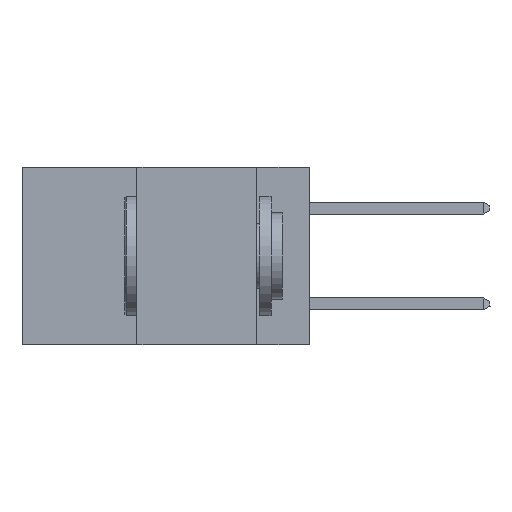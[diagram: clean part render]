
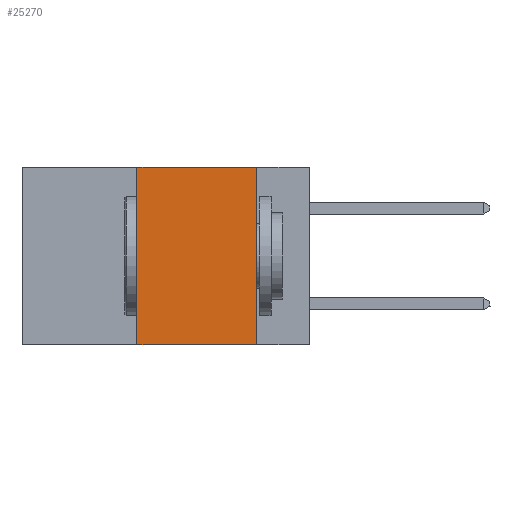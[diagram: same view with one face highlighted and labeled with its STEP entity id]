
A CAD part, left-side view. The second image highlights one B-rep face of the part: STEP entity #25270.
In plain terms, the highlighted planar face has unit normal (-1, 0, 0).
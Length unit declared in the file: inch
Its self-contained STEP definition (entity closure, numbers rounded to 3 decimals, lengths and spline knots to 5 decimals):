
#163 = DIRECTION ( 'NONE',  ( 0., 0., 1. ) ) ;
#1433 = VECTOR ( 'NONE', #27203, 39.37008 ) ;
#1575 = CARTESIAN_POINT ( 'NONE',  ( 0., 0.6, -0.37 ) ) ;
#2614 = ORIENTED_EDGE ( 'NONE', *, *, #15378, .F. ) ;
#3255 = EDGE_CURVE ( 'NONE', #10480, #33487, #26829, .T. ) ;
#4716 = VECTOR ( 'NONE', #163, 39.37008 ) ;
#5505 = FACE_OUTER_BOUND ( 'NONE', #15615, .T. ) ;
#6661 = EDGE_CURVE ( 'NONE', #14457, #33487, #10487, .T. ) ;
#7569 = DIRECTION ( 'NONE',  ( 1., 0., 0. ) ) ;
#8015 = CARTESIAN_POINT ( 'NONE',  ( 0., 0.6, 0. ) ) ;
#8068 = CARTESIAN_POINT ( 'NONE',  ( 0., 0.6, 0. ) ) ;
#10480 = VERTEX_POINT ( 'NONE', #25116 ) ;
#10487 = LINE ( 'NONE', #1575, #20457 ) ;
#12196 = EDGE_CURVE ( 'NONE', #14457, #17482, #30024, .T. ) ;
#14450 = LINE ( 'NONE', #8068, #27742 ) ;
#14457 = VERTEX_POINT ( 'NONE', #21364 ) ;
#15378 = EDGE_CURVE ( 'NONE', #17482, #10480, #14450, .T. ) ;
#15615 = EDGE_LOOP ( 'NONE', ( #22516, #2614, #18377, #18908 ) ) ;
#15893 = CARTESIAN_POINT ( 'NONE',  ( 0., 0.36, 0. ) ) ;
#17173 = CARTESIAN_POINT ( 'NONE',  ( 0., 0.36, 0. ) ) ;
#17429 = DIRECTION ( 'NONE',  ( 0., -1., 0. ) ) ;
#17482 = VERTEX_POINT ( 'NONE', #17173 ) ;
#18377 = ORIENTED_EDGE ( 'NONE', *, *, #12196, .F. ) ;
#18908 = ORIENTED_EDGE ( 'NONE', *, *, #6661, .T. ) ;
#20457 = VECTOR ( 'NONE', #31063, 39.37008 ) ;
#20846 = DIRECTION ( 'NONE',  ( 0., 0., -1. ) ) ;
#21364 = CARTESIAN_POINT ( 'NONE',  ( 0., 0.36, -0.37 ) ) ;
#21663 = CARTESIAN_POINT ( 'NONE',  ( 0., 0.11, 0. ) ) ;
#22516 = ORIENTED_EDGE ( 'NONE', *, *, #3255, .F. ) ;
#23502 = PLANE ( 'NONE',  #33424 ) ;
#25116 = CARTESIAN_POINT ( 'NONE',  ( 0., 0.11, 0. ) ) ;
#25270 = ADVANCED_FACE ( 'NONE', ( #5505 ), #23502, .F. ) ;
#26829 = LINE ( 'NONE', #21663, #1433 ) ;
#27203 = DIRECTION ( 'NONE',  ( 0., 0., -1. ) ) ;
#27742 = VECTOR ( 'NONE', #17429, 39.37008 ) ;
#30024 = LINE ( 'NONE', #15893, #4716 ) ;
#31063 = DIRECTION ( 'NONE',  ( 0., -1., 0. ) ) ;
#32485 = CARTESIAN_POINT ( 'NONE',  ( 0., 0.11, -0.37 ) ) ;
#33424 = AXIS2_PLACEMENT_3D ( 'NONE', #8015, #7569, #20846 ) ;
#33487 = VERTEX_POINT ( 'NONE', #32485 ) ;
